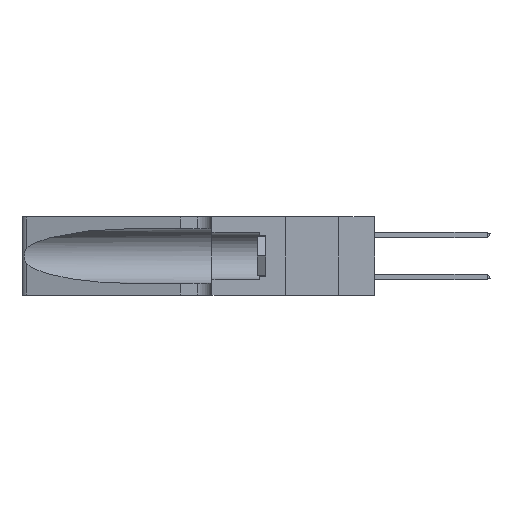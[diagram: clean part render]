
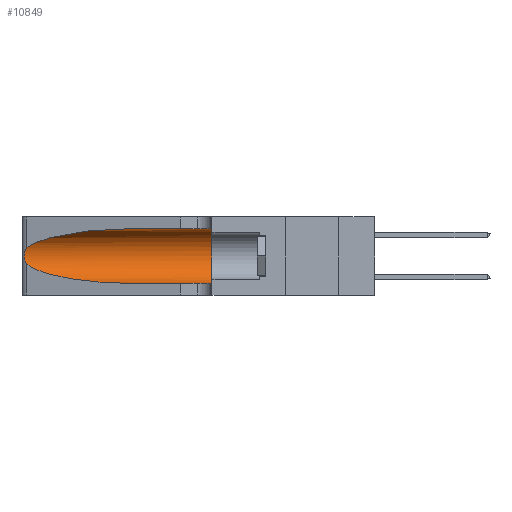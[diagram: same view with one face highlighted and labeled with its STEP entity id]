
A CAD part, left-side view. The second image highlights one B-rep face of the part: STEP entity #10849.
In plain terms, the highlighted cylindrical face has radius 3.308 mm (diameter 6.617 mm), a partial arc.
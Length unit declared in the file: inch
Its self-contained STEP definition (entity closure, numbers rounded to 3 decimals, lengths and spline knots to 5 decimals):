
#39 = EDGE_CURVE ( 'NONE', #28640, #28751, #13280, .T. ) ;
#268 = CARTESIAN_POINT ( 'NONE',  ( 0.18966, 0.96281, 0.05475 ) ) ;
#1201 = DIRECTION ( 'NONE',  ( 0., 0., -1. ) ) ;
#1348 = DIRECTION ( 'NONE',  ( 0., -1., 0. ) ) ;
#2031 = CARTESIAN_POINT ( 'NONE',  ( 0.25487, 1.22718, 0.14631 ) ) ;
#2032 = CARTESIAN_POINT ( 'NONE',  ( 0.25487, 1.22718, 0.22369 ) ) ;
#3558 = EDGE_CURVE ( 'NONE', #28640, #31572, #25491, .T. ) ;
#4489 = ORIENTED_EDGE ( 'NONE', *, *, #40127, .T. ) ;
#5392 = CARTESIAN_POINT ( 'NONE',  ( 0.25639, 1.23184, 0.21858 ) ) ;
#6276 = CARTESIAN_POINT ( 'NONE',  ( 0.25487, 1.22718, 0.22369 ) ) ;
#8374 = EDGE_LOOP ( 'NONE', ( #17492, #4489, #27173, #39397, #38486, #35029 ) ) ;
#8845 = CARTESIAN_POINT ( 'NONE',  ( 0.25854, 1.2359, 0.20912 ) ) ;
#9639 = VERTEX_POINT ( 'NONE', #24788 ) ;
#10511 = DIRECTION ( 'NONE',  ( 0., 1., 0. ) ) ;
#10849 = ADVANCED_FACE ( 'NONE', ( #41296 ), #15045, .F. ) ;
#12192 = CARTESIAN_POINT ( 'NONE',  ( 0.26075, 1.23896, 0.19203 ) ) ;
#13280 =( BOUNDED_CURVE ( )  B_SPLINE_CURVE ( 3, ( #26198, #42541, #16260, #6276 ),
 .UNSPECIFIED., .F., .F. ) 
 B_SPLINE_CURVE_WITH_KNOTS ( ( 4, 4 ),
 ( 1.5708, 2.84003 ),
 .UNSPECIFIED. ) 
 CURVE ( )  GEOMETRIC_REPRESENTATION_ITEM ( )  RATIONAL_B_SPLINE_CURVE ( ( 1., 0.87, 0.87, 1. ) ) 
 REPRESENTATION_ITEM ( '' )  );
#13905 = DIRECTION ( 'NONE',  ( 0., -1., 0. ) ) ;
#14311 = EDGE_CURVE ( 'NONE', #31572, #9639, #29256, .T. ) ;
#14595 = B_SPLINE_CURVE_WITH_KNOTS ( 'NONE', 3,
 ( #41723, #18785, #5392, #28655, #8845, #31982, #12192, #35276, #15556, #38582, #18923, #41873, #22207, #2031 ),
 .UNSPECIFIED., .F., .F.,
 ( 4, 2, 2, 2, 2, 2, 4 ),
 ( 0., 0.00027, 0.00053, 0.00107, 0.0016, 0.00187, 0.00214 ),
 .UNSPECIFIED. ) ;
#14973 = CARTESIAN_POINT ( 'NONE',  ( 0.1305, 0.72297, 0.05475 ) ) ;
#15045 = CYLINDRICAL_SURFACE ( 'NONE', #31829, 0.13025 ) ;
#15556 = CARTESIAN_POINT ( 'NONE',  ( 0.26017, 1.23833, 0.17102 ) ) ;
#16109 = CARTESIAN_POINT ( 'NONE',  ( 0.25487, 1.22718, 0.14631 ) ) ;
#16260 = CARTESIAN_POINT ( 'NONE',  ( 0.2373, 1.15595, 0.28018 ) ) ;
#16750 = VECTOR ( 'NONE', #13905, 39.37008 ) ;
#17203 = CARTESIAN_POINT ( 'NONE',  ( 0.25487, 1.22718, 0.14631 ) ) ;
#17492 = ORIENTED_EDGE ( 'NONE', *, *, #39, .T. ) ;
#18785 = CARTESIAN_POINT ( 'NONE',  ( 0.25555, 1.22994, 0.2215 ) ) ;
#18923 = CARTESIAN_POINT ( 'NONE',  ( 0.25789, 1.23486, 0.15765 ) ) ;
#22207 = CARTESIAN_POINT ( 'NONE',  ( 0.25555, 1.22993, 0.14849 ) ) ;
#23812 = CARTESIAN_POINT ( 'NONE',  ( 0.1305, 0.72297, 0.05475 ) ) ;
#24645 = VECTOR ( 'NONE', #32738, 39.37008 ) ;
#24788 = CARTESIAN_POINT ( 'NONE',  ( 0.1305, 0.35, 0.05475 ) ) ;
#25491 = LINE ( 'NONE', #33495, #16750 ) ;
#26198 = CARTESIAN_POINT ( 'NONE',  ( 0.1305, 0.72297, 0.31525 ) ) ;
#27173 = ORIENTED_EDGE ( 'NONE', *, *, #37112, .T. ) ;
#28134 = CARTESIAN_POINT ( 'NONE',  ( 0.1305, 0.35, 0.31525 ) ) ;
#28629 = VERTEX_POINT ( 'NONE', #14973 ) ;
#28640 = VERTEX_POINT ( 'NONE', #38005 ) ;
#28655 = CARTESIAN_POINT ( 'NONE',  ( 0.25787, 1.23484, 0.2124 ) ) ;
#28751 = VERTEX_POINT ( 'NONE', #2032 ) ;
#29256 = CIRCLE ( 'NONE', #34944, 0.13025 ) ;
#29431 = CARTESIAN_POINT ( 'NONE',  ( 0.1305, 1.61858, 0.05475 ) ) ;
#29754 = EDGE_CURVE ( 'NONE', #28629, #9639, #32352, .T. ) ;
#29960 =( BOUNDED_CURVE ( )  B_SPLINE_CURVE ( 3, ( #17203, #36863, #268, #23812 ),
 .UNSPECIFIED., .F., .F. ) 
 B_SPLINE_CURVE_WITH_KNOTS ( ( 4, 4 ),
 ( 3.44316, 4.71239 ),
 .UNSPECIFIED. ) 
 CURVE ( )  GEOMETRIC_REPRESENTATION_ITEM ( )  RATIONAL_B_SPLINE_CURVE ( ( 1., 0.87, 0.87, 1. ) ) 
 REPRESENTATION_ITEM ( '' )  );
#30316 = CARTESIAN_POINT ( 'NONE',  ( 0.1305, 0.35, 0.185 ) ) ;
#31572 = VERTEX_POINT ( 'NONE', #28134 ) ;
#31829 = AXIS2_PLACEMENT_3D ( 'NONE', #34596, #1348, #1201 ) ;
#31982 = CARTESIAN_POINT ( 'NONE',  ( 0.26018, 1.23835, 0.19895 ) ) ;
#32352 = LINE ( 'NONE', #29431, #24645 ) ;
#32738 = DIRECTION ( 'NONE',  ( 0., -1., 0. ) ) ;
#33495 = CARTESIAN_POINT ( 'NONE',  ( 0.1305, 1.61858, 0.31525 ) ) ;
#33602 = DIRECTION ( 'NONE',  ( 0., 0., 1. ) ) ;
#34427 = VERTEX_POINT ( 'NONE', #16109 ) ;
#34596 = CARTESIAN_POINT ( 'NONE',  ( 0.1305, 1.61858, 0.185 ) ) ;
#34944 = AXIS2_PLACEMENT_3D ( 'NONE', #30316, #10511, #33602 ) ;
#35029 = ORIENTED_EDGE ( 'NONE', *, *, #3558, .F. ) ;
#35276 = CARTESIAN_POINT ( 'NONE',  ( 0.26075, 1.23896, 0.178 ) ) ;
#36863 = CARTESIAN_POINT ( 'NONE',  ( 0.2373, 1.15595, 0.08982 ) ) ;
#37112 = EDGE_CURVE ( 'NONE', #34427, #28629, #29960, .T. ) ;
#38005 = CARTESIAN_POINT ( 'NONE',  ( 0.1305, 0.72297, 0.31525 ) ) ;
#38486 = ORIENTED_EDGE ( 'NONE', *, *, #14311, .F. ) ;
#38582 = CARTESIAN_POINT ( 'NONE',  ( 0.25856, 1.23593, 0.16098 ) ) ;
#39397 = ORIENTED_EDGE ( 'NONE', *, *, #29754, .T. ) ;
#40127 = EDGE_CURVE ( 'NONE', #28751, #34427, #14595, .T. ) ;
#41296 = FACE_OUTER_BOUND ( 'NONE', #8374, .T. ) ;
#41723 = CARTESIAN_POINT ( 'NONE',  ( 0.25487, 1.22718, 0.22369 ) ) ;
#41873 = CARTESIAN_POINT ( 'NONE',  ( 0.25639, 1.23186, 0.15144 ) ) ;
#42541 = CARTESIAN_POINT ( 'NONE',  ( 0.18966, 0.96281, 0.31525 ) ) ;
